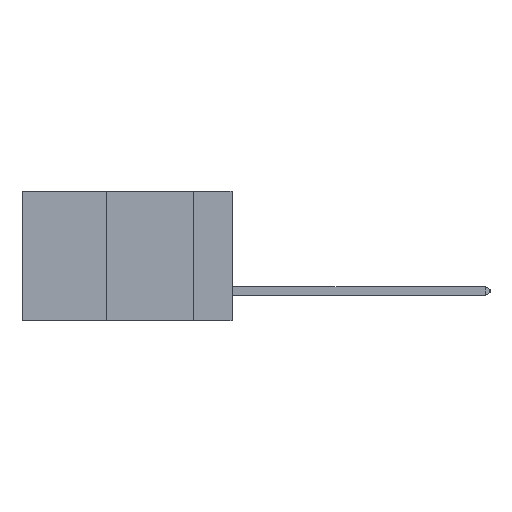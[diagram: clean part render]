
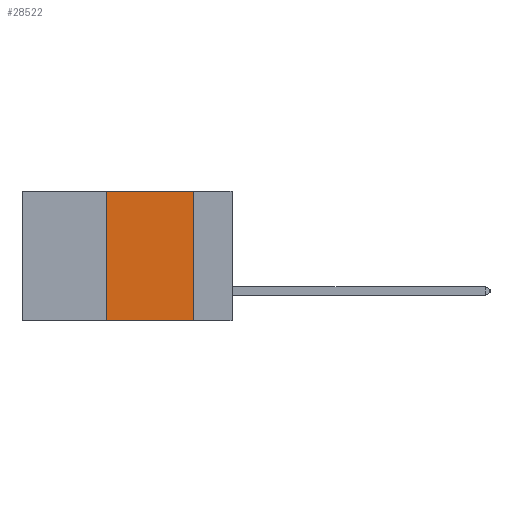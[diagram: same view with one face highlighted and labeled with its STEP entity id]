
A CAD part, left-side view. The second image highlights one B-rep face of the part: STEP entity #28522.
In plain terms, the highlighted planar face has unit normal (-1, 0, 0).
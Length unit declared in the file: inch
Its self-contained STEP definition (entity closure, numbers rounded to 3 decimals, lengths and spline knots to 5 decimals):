
#1008 = EDGE_CURVE ( 'NONE', #18774, #2032, #9152, .T. ) ;
#2032 = VERTEX_POINT ( 'NONE', #14495 ) ;
#2818 = EDGE_CURVE ( 'NONE', #2032, #17874, #6934, .T. ) ;
#3083 = VECTOR ( 'NONE', #14801, 39.37008 ) ;
#4700 = CARTESIAN_POINT ( 'NONE',  ( 0., 0.6, -0.37 ) ) ;
#4904 = ORIENTED_EDGE ( 'NONE', *, *, #1008, .F. ) ;
#6934 = LINE ( 'NONE', #25539, #23969 ) ;
#7086 = DIRECTION ( 'NONE',  ( 0., 0., -1. ) ) ;
#7167 = VECTOR ( 'NONE', #22192, 39.37008 ) ;
#9152 = LINE ( 'NONE', #14904, #3083 ) ;
#9882 = PLANE ( 'NONE',  #22780 ) ;
#10241 = ORIENTED_EDGE ( 'NONE', *, *, #2818, .F. ) ;
#10505 = CARTESIAN_POINT ( 'NONE',  ( 0., 0.36, 0. ) ) ;
#12156 = DIRECTION ( 'NONE',  ( 1., 0., 0. ) ) ;
#12921 = LINE ( 'NONE', #4700, #23303 ) ;
#14495 = CARTESIAN_POINT ( 'NONE',  ( 0., 0.11, 0. ) ) ;
#14801 = DIRECTION ( 'NONE',  ( 0., -1., 0. ) ) ;
#14879 = EDGE_CURVE ( 'NONE', #19093, #18774, #19111, .T. ) ;
#14904 = CARTESIAN_POINT ( 'NONE',  ( 0., 0.6, 0. ) ) ;
#17600 = ORIENTED_EDGE ( 'NONE', *, *, #14879, .F. ) ;
#17874 = VERTEX_POINT ( 'NONE', #19337 ) ;
#18774 = VERTEX_POINT ( 'NONE', #10505 ) ;
#19093 = VERTEX_POINT ( 'NONE', #27001 ) ;
#19111 = LINE ( 'NONE', #28827, #7167 ) ;
#19337 = CARTESIAN_POINT ( 'NONE',  ( 0., 0.11, -0.37 ) ) ;
#21923 = EDGE_LOOP ( 'NONE', ( #10241, #4904, #17600, #23432 ) ) ;
#22192 = DIRECTION ( 'NONE',  ( 0., 0., 1. ) ) ;
#22619 = DIRECTION ( 'NONE',  ( 0., -1., 0. ) ) ;
#22780 = AXIS2_PLACEMENT_3D ( 'NONE', #25361, #12156, #27598 ) ;
#22940 = EDGE_CURVE ( 'NONE', #19093, #17874, #12921, .T. ) ;
#23303 = VECTOR ( 'NONE', #22619, 39.37008 ) ;
#23432 = ORIENTED_EDGE ( 'NONE', *, *, #22940, .T. ) ;
#23969 = VECTOR ( 'NONE', #7086, 39.37008 ) ;
#24570 = FACE_OUTER_BOUND ( 'NONE', #21923, .T. ) ;
#25361 = CARTESIAN_POINT ( 'NONE',  ( 0., 0.6, 0. ) ) ;
#25539 = CARTESIAN_POINT ( 'NONE',  ( 0., 0.11, 0. ) ) ;
#27001 = CARTESIAN_POINT ( 'NONE',  ( 0., 0.36, -0.37 ) ) ;
#27598 = DIRECTION ( 'NONE',  ( 0., 0., -1. ) ) ;
#28522 = ADVANCED_FACE ( 'NONE', ( #24570 ), #9882, .F. ) ;
#28827 = CARTESIAN_POINT ( 'NONE',  ( 0., 0.36, 0. ) ) ;
